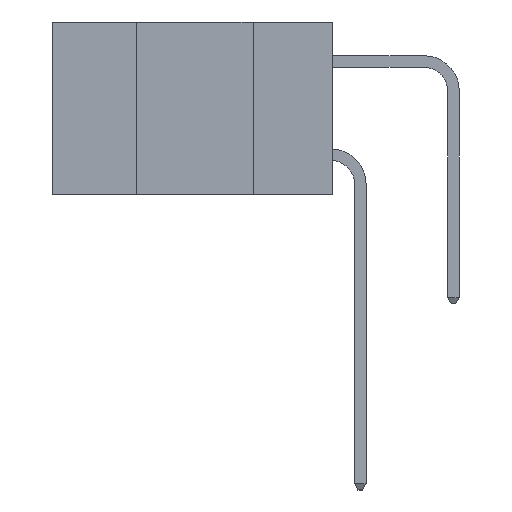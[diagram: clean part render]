
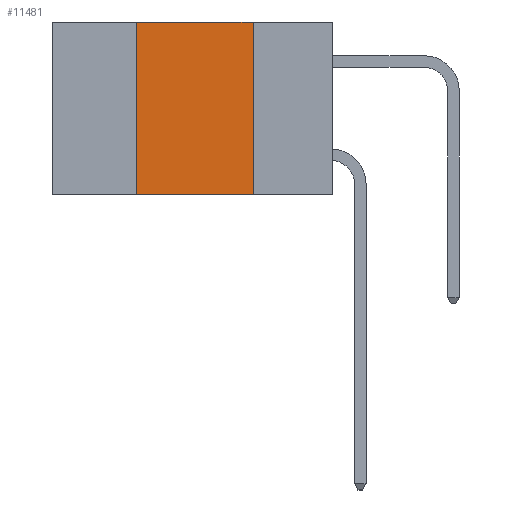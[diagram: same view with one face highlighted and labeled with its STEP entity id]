
A CAD part, left-side view. The second image highlights one B-rep face of the part: STEP entity #11481.
In plain terms, the highlighted planar face has unit normal (-1, 0, 0).
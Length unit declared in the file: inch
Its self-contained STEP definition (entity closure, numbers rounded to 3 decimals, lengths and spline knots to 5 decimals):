
#194 = CARTESIAN_POINT ( 'NONE',  ( 0., 0.17, -0.37 ) ) ;
#559 = LINE ( 'NONE', #3683, #3892 ) ;
#1390 = LINE ( 'NONE', #12518, #14669 ) ;
#1778 = VERTEX_POINT ( 'NONE', #12562 ) ;
#1789 = EDGE_CURVE ( 'NONE', #7439, #1778, #1390, .T. ) ;
#2462 = CARTESIAN_POINT ( 'NONE',  ( 0., 0.17, 0. ) ) ;
#3478 = DIRECTION ( 'NONE',  ( 0., -1., 0. ) ) ;
#3527 = CARTESIAN_POINT ( 'NONE',  ( 0., 0.42, -0.37 ) ) ;
#3683 = CARTESIAN_POINT ( 'NONE',  ( 0., 0.6, 0. ) ) ;
#3892 = VECTOR ( 'NONE', #3478, 39.37008 ) ;
#4161 = EDGE_CURVE ( 'NONE', #7439, #6886, #16190, .T. ) ;
#4857 = VECTOR ( 'NONE', #9661, 39.37008 ) ;
#5884 = VECTOR ( 'NONE', #8092, 39.37008 ) ;
#6886 = VERTEX_POINT ( 'NONE', #9591 ) ;
#7439 = VERTEX_POINT ( 'NONE', #3527 ) ;
#7876 = CARTESIAN_POINT ( 'NONE',  ( 0., 0.6, -0.37 ) ) ;
#8092 = DIRECTION ( 'NONE',  ( 0., -1., 0. ) ) ;
#8109 = ORIENTED_EDGE ( 'NONE', *, *, #11914, .F. ) ;
#8216 = ORIENTED_EDGE ( 'NONE', *, *, #1789, .F. ) ;
#9591 = CARTESIAN_POINT ( 'NONE',  ( 0., 0.17, -0.37 ) ) ;
#9661 = DIRECTION ( 'NONE',  ( 0., 0., -1. ) ) ;
#11481 = ADVANCED_FACE ( 'NONE', ( #11682 ), #12881, .F. ) ;
#11682 = FACE_OUTER_BOUND ( 'NONE', #14741, .T. ) ;
#11803 = DIRECTION ( 'NONE',  ( 0., 0., 1. ) ) ;
#11914 = EDGE_CURVE ( 'NONE', #1778, #14000, #559, .T. ) ;
#12518 = CARTESIAN_POINT ( 'NONE',  ( 0., 0.42, -0.37 ) ) ;
#12562 = CARTESIAN_POINT ( 'NONE',  ( 0., 0.42, 0. ) ) ;
#12785 = DIRECTION ( 'NONE',  ( 0., 0., -1. ) ) ;
#12823 = DIRECTION ( 'NONE',  ( 1., 0., 0. ) ) ;
#12881 = PLANE ( 'NONE',  #15424 ) ;
#13044 = CARTESIAN_POINT ( 'NONE',  ( 0., 0.6, 0. ) ) ;
#14000 = VERTEX_POINT ( 'NONE', #2462 ) ;
#14231 = ORIENTED_EDGE ( 'NONE', *, *, #14855, .F. ) ;
#14669 = VECTOR ( 'NONE', #11803, 39.37008 ) ;
#14741 = EDGE_LOOP ( 'NONE', ( #14231, #8109, #8216, #16644 ) ) ;
#14830 = LINE ( 'NONE', #194, #4857 ) ;
#14855 = EDGE_CURVE ( 'NONE', #14000, #6886, #14830, .T. ) ;
#15424 = AXIS2_PLACEMENT_3D ( 'NONE', #13044, #12823, #12785 ) ;
#16190 = LINE ( 'NONE', #7876, #5884 ) ;
#16644 = ORIENTED_EDGE ( 'NONE', *, *, #4161, .T. ) ;
